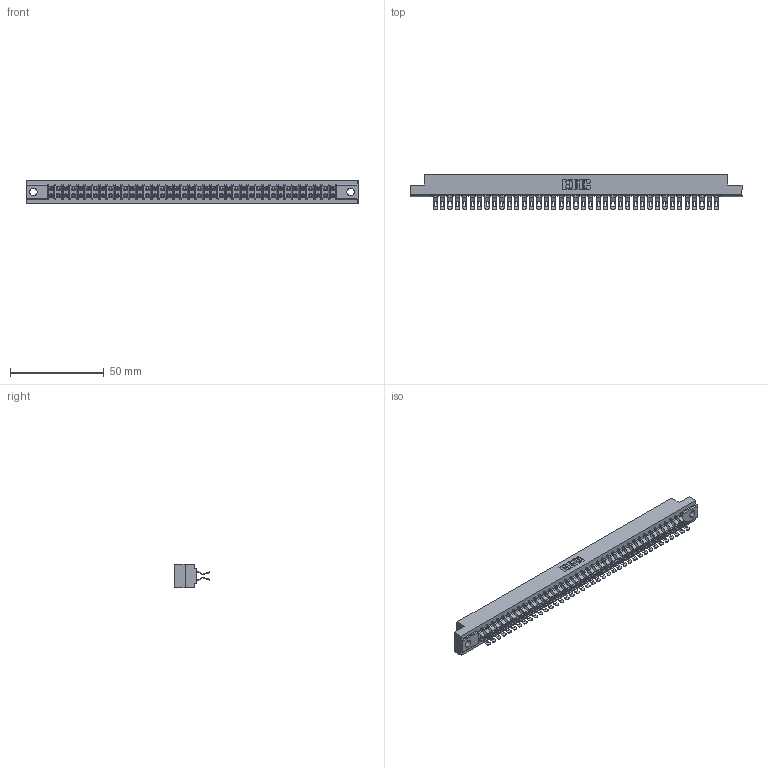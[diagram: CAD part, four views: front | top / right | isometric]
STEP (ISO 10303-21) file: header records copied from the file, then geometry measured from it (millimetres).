
FILE_DESCRIPTION (( 'STEP AP203' ), '1' );
FILE_NAME ('357-078-455-202.STEP', '2020-10-04T13:27:43', ( '' ), ( '' ), 'SwSTEP 2.0', 'SolidWorks 2020', '' );
FILE_SCHEMA (( 'CONFIG_CONTROL_DESIGN' ));
Length unit declared in the file: inch
Products named in the file (3): 307 Part_.128 Dia Mounting Holes; 357-078-455-202; 307-290-001_555
Assembly tree (79 placements, depth 2):
  357-078-455-202
    307 Part_.128 Dia Mounting Holes
    307-290-001_555  x78
Bounding box: 177.55 x 18.75 x 12.7 mm (x, y, z)
Volume: 19003.2 mm3; surface area: 24282.4 mm2
Topology: 79 solids, 79 shells, 4916 faces, 14441 edges, 9414 vertices
Faces by surface type: plane 2722, cylinder 2114, sphere 80
Entity records: 35591 total; most frequent: CARTESIAN_POINT 5827, ORIENTED_EDGE 5776, DIRECTION 5716, EDGE_CURVE 2888, LINE 2202, VECTOR 2202, VERTEX_POINT 1868, AXIS2_PLACEMENT_3D 1757
